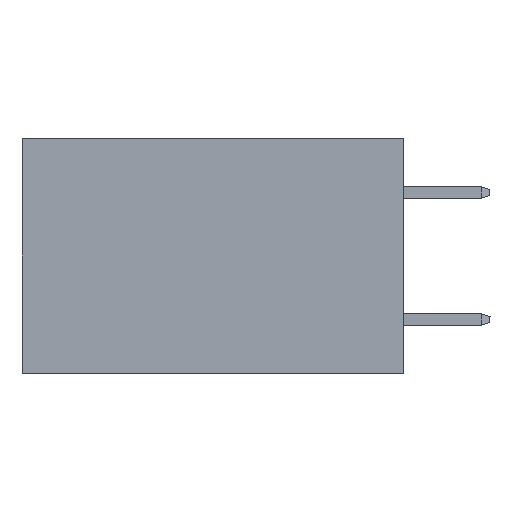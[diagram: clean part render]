
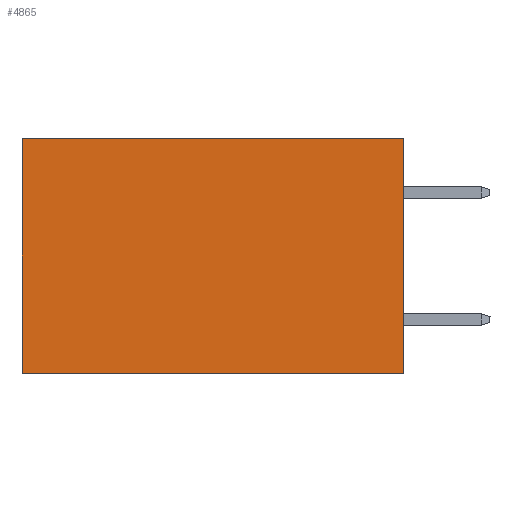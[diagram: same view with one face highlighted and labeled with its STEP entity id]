
A CAD part, left-side view. The second image highlights one B-rep face of the part: STEP entity #4865.
In plain terms, the highlighted planar face has unit normal (-1, 0, 0).
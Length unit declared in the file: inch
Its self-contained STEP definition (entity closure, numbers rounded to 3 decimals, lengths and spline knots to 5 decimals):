
#956 = EDGE_CURVE ( 'NONE', #15886, #12270, #10830, .T. ) ;
#966 = CARTESIAN_POINT ( 'NONE',  ( 0.2875, 0., -0.37 ) ) ;
#1214 = LINE ( 'NONE', #8253, #16052 ) ;
#1618 = PLANE ( 'NONE',  #17160 ) ;
#3059 = EDGE_LOOP ( 'NONE', ( #15462, #12630, #4070, #10407 ) ) ;
#3392 = CARTESIAN_POINT ( 'NONE',  ( 0.2875, 0., 0. ) ) ;
#3785 = LINE ( 'NONE', #9324, #8107 ) ;
#3865 = EDGE_CURVE ( 'NONE', #9228, #15886, #7097, .T. ) ;
#3949 = CARTESIAN_POINT ( 'NONE',  ( 0.2875, 0., -0.37 ) ) ;
#4070 = ORIENTED_EDGE ( 'NONE', *, *, #3865, .F. ) ;
#4865 = ADVANCED_FACE ( 'NONE', ( #8493 ), #1618, .F. ) ;
#5646 = CARTESIAN_POINT ( 'NONE',  ( 0.2875, 0., 0. ) ) ;
#6042 = EDGE_CURVE ( 'NONE', #12488, #12270, #1214, .T. ) ;
#6556 = DIRECTION ( 'NONE',  ( 0., 0., -1. ) ) ;
#7097 = LINE ( 'NONE', #5646, #14888 ) ;
#7669 = CARTESIAN_POINT ( 'NONE',  ( 0.2875, 0.6, -0.37 ) ) ;
#8107 = VECTOR ( 'NONE', #14824, 39.37008 ) ;
#8253 = CARTESIAN_POINT ( 'NONE',  ( 0.2875, 0.6, 0. ) ) ;
#8493 = FACE_OUTER_BOUND ( 'NONE', #3059, .T. ) ;
#9017 = CARTESIAN_POINT ( 'NONE',  ( 0.2875, 0., 0. ) ) ;
#9126 = DIRECTION ( 'NONE',  ( 0., 1., 0. ) ) ;
#9228 = VERTEX_POINT ( 'NONE', #3392 ) ;
#9324 = CARTESIAN_POINT ( 'NONE',  ( 0.2875, 0., 0. ) ) ;
#10407 = ORIENTED_EDGE ( 'NONE', *, *, #12038, .T. ) ;
#10459 = CARTESIAN_POINT ( 'NONE',  ( 0.2875, 0.6, 0. ) ) ;
#10830 = LINE ( 'NONE', #3949, #14399 ) ;
#12038 = EDGE_CURVE ( 'NONE', #9228, #12488, #3785, .T. ) ;
#12270 = VERTEX_POINT ( 'NONE', #7669 ) ;
#12488 = VERTEX_POINT ( 'NONE', #10459 ) ;
#12630 = ORIENTED_EDGE ( 'NONE', *, *, #956, .F. ) ;
#13069 = DIRECTION ( 'NONE',  ( 1., 0., 0. ) ) ;
#14055 = DIRECTION ( 'NONE',  ( 0., 0., -1. ) ) ;
#14399 = VECTOR ( 'NONE', #9126, 39.37008 ) ;
#14824 = DIRECTION ( 'NONE',  ( 0., 1., 0. ) ) ;
#14888 = VECTOR ( 'NONE', #14055, 39.37008 ) ;
#15462 = ORIENTED_EDGE ( 'NONE', *, *, #6042, .T. ) ;
#15886 = VERTEX_POINT ( 'NONE', #966 ) ;
#16052 = VECTOR ( 'NONE', #17624, 39.37008 ) ;
#17160 = AXIS2_PLACEMENT_3D ( 'NONE', #9017, #13069, #6556 ) ;
#17624 = DIRECTION ( 'NONE',  ( 0., 0., -1. ) ) ;
